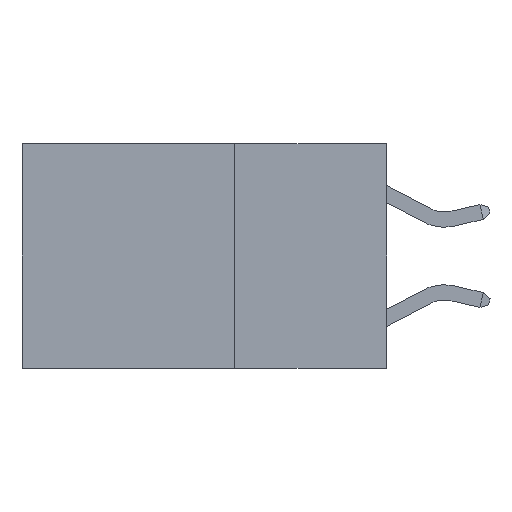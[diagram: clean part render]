
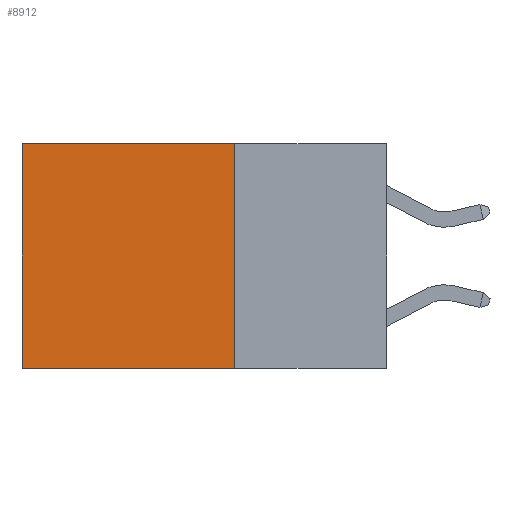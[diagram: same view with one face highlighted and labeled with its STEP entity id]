
A CAD part, left-side view. The second image highlights one B-rep face of the part: STEP entity #8912.
In plain terms, the highlighted planar face has unit normal (-1, 0, 0).
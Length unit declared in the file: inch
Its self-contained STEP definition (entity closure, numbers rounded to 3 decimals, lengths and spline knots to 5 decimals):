
#2155 = VECTOR ( 'NONE', #10827, 39.37008 ) ;
#2240 = ORIENTED_EDGE ( 'NONE', *, *, #17144, .F. ) ;
#4309 = EDGE_LOOP ( 'NONE', ( #6455, #14768, #2240, #12715 ) ) ;
#5394 = CARTESIAN_POINT ( 'NONE',  ( 0.2625, 0.25, 0. ) ) ;
#5504 = LINE ( 'NONE', #24669, #20803 ) ;
#6455 = ORIENTED_EDGE ( 'NONE', *, *, #20986, .T. ) ;
#6649 = VERTEX_POINT ( 'NONE', #18107 ) ;
#7122 = CARTESIAN_POINT ( 'NONE',  ( 0.2625, 0.6, 0. ) ) ;
#7195 = FACE_OUTER_BOUND ( 'NONE', #4309, .T. ) ;
#7553 = PLANE ( 'NONE',  #13370 ) ;
#8912 = ADVANCED_FACE ( 'NONE', ( #7195 ), #7553, .F. ) ;
#9594 = DIRECTION ( 'NONE',  ( 1., 0., 0. ) ) ;
#10827 = DIRECTION ( 'NONE',  ( 0., 0., -1. ) ) ;
#10932 = DIRECTION ( 'NONE',  ( 0., 1., 0. ) ) ;
#11065 = DIRECTION ( 'NONE',  ( 0., 0., -1. ) ) ;
#12602 = LINE ( 'NONE', #5394, #17905 ) ;
#12715 = ORIENTED_EDGE ( 'NONE', *, *, #16656, .T. ) ;
#13370 = AXIS2_PLACEMENT_3D ( 'NONE', #21460, #9594, #23368 ) ;
#14009 = EDGE_CURVE ( 'NONE', #6649, #22462, #5504, .T. ) ;
#14768 = ORIENTED_EDGE ( 'NONE', *, *, #14009, .F. ) ;
#15435 = LINE ( 'NONE', #24798, #20716 ) ;
#16656 = EDGE_CURVE ( 'NONE', #23254, #20516, #12602, .T. ) ;
#17144 = EDGE_CURVE ( 'NONE', #23254, #6649, #22681, .T. ) ;
#17354 = CARTESIAN_POINT ( 'NONE',  ( 0.2625, 0.6, -0.37 ) ) ;
#17382 = DIRECTION ( 'NONE',  ( 0., 1., 0. ) ) ;
#17905 = VECTOR ( 'NONE', #17382, 39.37008 ) ;
#18107 = CARTESIAN_POINT ( 'NONE',  ( 0.2625, 0.25, -0.37 ) ) ;
#20516 = VERTEX_POINT ( 'NONE', #7122 ) ;
#20716 = VECTOR ( 'NONE', #11065, 39.37008 ) ;
#20803 = VECTOR ( 'NONE', #10932, 39.37008 ) ;
#20986 = EDGE_CURVE ( 'NONE', #20516, #22462, #15435, .T. ) ;
#21460 = CARTESIAN_POINT ( 'NONE',  ( 0.2625, 0.25, 0. ) ) ;
#22462 = VERTEX_POINT ( 'NONE', #17354 ) ;
#22681 = LINE ( 'NONE', #24574, #2155 ) ;
#23254 = VERTEX_POINT ( 'NONE', #23603 ) ;
#23368 = DIRECTION ( 'NONE',  ( 0., 0., -1. ) ) ;
#23603 = CARTESIAN_POINT ( 'NONE',  ( 0.2625, 0.25, 0. ) ) ;
#24574 = CARTESIAN_POINT ( 'NONE',  ( 0.2625, 0.25, 0. ) ) ;
#24669 = CARTESIAN_POINT ( 'NONE',  ( 0.2625, 0.25, -0.37 ) ) ;
#24798 = CARTESIAN_POINT ( 'NONE',  ( 0.2625, 0.6, 0. ) ) ;
